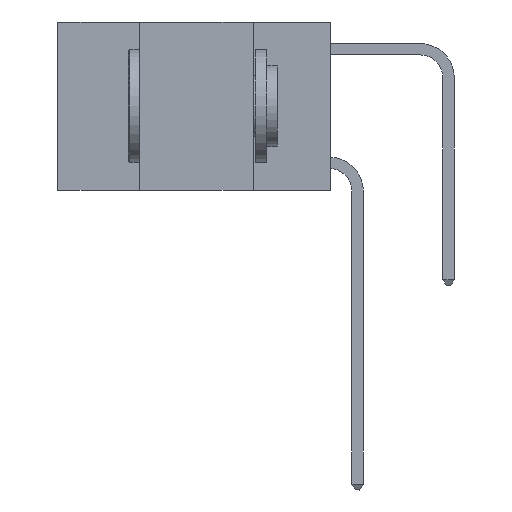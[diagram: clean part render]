
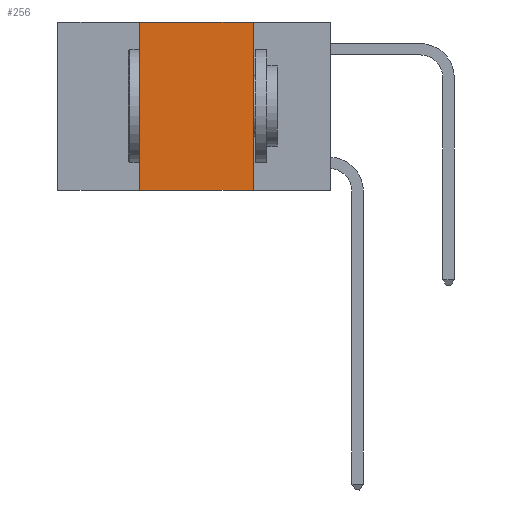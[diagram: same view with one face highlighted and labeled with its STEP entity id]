
A CAD part, left-side view. The second image highlights one B-rep face of the part: STEP entity #256.
In plain terms, the highlighted planar face has unit normal (-1, 0, 0).
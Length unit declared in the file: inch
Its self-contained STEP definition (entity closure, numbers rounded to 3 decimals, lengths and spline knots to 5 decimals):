
#256 = ADVANCED_FACE ( 'NONE', ( #2609 ), #14112, .F. ) ;
#1143 = DIRECTION ( 'NONE',  ( 0., -1., 0. ) ) ;
#1716 = ORIENTED_EDGE ( 'NONE', *, *, #10080, .F. ) ;
#2176 = CARTESIAN_POINT ( 'NONE',  ( 0., 0.17, 0. ) ) ;
#2609 = FACE_OUTER_BOUND ( 'NONE', #5410, .T. ) ;
#2650 = VECTOR ( 'NONE', #12887, 39.37008 ) ;
#4871 = DIRECTION ( 'NONE',  ( 0., 0., -1. ) ) ;
#4876 = ORIENTED_EDGE ( 'NONE', *, *, #7117, .F. ) ;
#4946 = CARTESIAN_POINT ( 'NONE',  ( 0., 0.42, -0.37 ) ) ;
#5237 = CARTESIAN_POINT ( 'NONE',  ( 0., 0.42, 0. ) ) ;
#5400 = CARTESIAN_POINT ( 'NONE',  ( 0., 0.6, -0.37 ) ) ;
#5410 = EDGE_LOOP ( 'NONE', ( #9628, #1716, #4876, #6243 ) ) ;
#5787 = VECTOR ( 'NONE', #4871, 39.37008 ) ;
#6243 = ORIENTED_EDGE ( 'NONE', *, *, #15823, .T. ) ;
#6312 = VECTOR ( 'NONE', #9624, 39.37008 ) ;
#7117 = EDGE_CURVE ( 'NONE', #17127, #8234, #10281, .T. ) ;
#7167 = LINE ( 'NONE', #19193, #18577 ) ;
#8234 = VERTEX_POINT ( 'NONE', #17795 ) ;
#8445 = EDGE_CURVE ( 'NONE', #19046, #10143, #18139, .T. ) ;
#9233 = AXIS2_PLACEMENT_3D ( 'NONE', #14735, #14582, #14445 ) ;
#9624 = DIRECTION ( 'NONE',  ( 0., 0., 1. ) ) ;
#9628 = ORIENTED_EDGE ( 'NONE', *, *, #8445, .F. ) ;
#10080 = EDGE_CURVE ( 'NONE', #8234, #19046, #7167, .T. ) ;
#10143 = VERTEX_POINT ( 'NONE', #10396 ) ;
#10281 = LINE ( 'NONE', #5237, #6312 ) ;
#10396 = CARTESIAN_POINT ( 'NONE',  ( 0., 0.17, -0.37 ) ) ;
#10675 = LINE ( 'NONE', #5400, #2650 ) ;
#10845 = CARTESIAN_POINT ( 'NONE',  ( 0., 0.17, 0. ) ) ;
#12887 = DIRECTION ( 'NONE',  ( 0., -1., 0. ) ) ;
#14112 = PLANE ( 'NONE',  #9233 ) ;
#14445 = DIRECTION ( 'NONE',  ( 0., 0., -1. ) ) ;
#14582 = DIRECTION ( 'NONE',  ( 1., 0., 0. ) ) ;
#14735 = CARTESIAN_POINT ( 'NONE',  ( 0., 0.6, 0. ) ) ;
#15823 = EDGE_CURVE ( 'NONE', #17127, #10143, #10675, .T. ) ;
#17127 = VERTEX_POINT ( 'NONE', #4946 ) ;
#17795 = CARTESIAN_POINT ( 'NONE',  ( 0., 0.42, 0. ) ) ;
#18139 = LINE ( 'NONE', #10845, #5787 ) ;
#18577 = VECTOR ( 'NONE', #1143, 39.37008 ) ;
#19046 = VERTEX_POINT ( 'NONE', #2176 ) ;
#19193 = CARTESIAN_POINT ( 'NONE',  ( 0., 0.6, 0. ) ) ;
